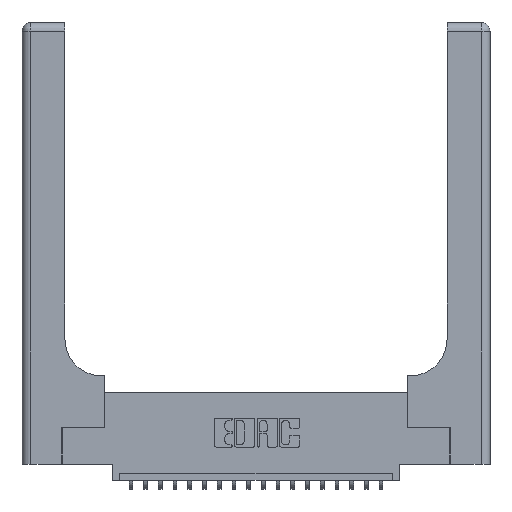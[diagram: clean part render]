
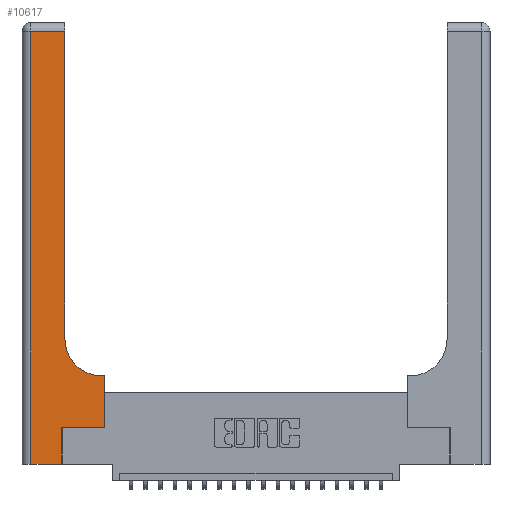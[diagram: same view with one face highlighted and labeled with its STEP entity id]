
A CAD part, top view. The second image highlights one B-rep face of the part: STEP entity #10617.
In plain terms, the highlighted planar face has unit normal (0, 0, 1).
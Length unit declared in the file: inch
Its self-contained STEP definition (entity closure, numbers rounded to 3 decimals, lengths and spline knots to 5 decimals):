
#414 = CARTESIAN_POINT ( 'NONE',  ( 0.2915, 0.85, 0.37 ) ) ;
#464 = CARTESIAN_POINT ( 'NONE',  ( 0., 3., 0.37 ) ) ;
#840 = VERTEX_POINT ( 'NONE', #6834 ) ;
#920 = VERTEX_POINT ( 'NONE', #7125 ) ;
#981 = EDGE_CURVE ( 'NONE', #17231, #18543, #9277, .T. ) ;
#1384 = EDGE_CURVE ( 'NONE', #18543, #18595, #11652, .T. ) ;
#2075 = CARTESIAN_POINT ( 'NONE',  ( 0.5415, 0.85, 0.37 ) ) ;
#2097 = CARTESIAN_POINT ( 'NONE',  ( 0.269, 0., 0.37 ) ) ;
#2369 = DIRECTION ( 'NONE',  ( 0., 1., 0. ) ) ;
#2375 = PLANE ( 'NONE',  #16137 ) ;
#2440 = EDGE_CURVE ( 'NONE', #20743, #15297, #5850, .T. ) ;
#2452 = AXIS2_PLACEMENT_3D ( 'NONE', #2075, #9241, #14116 ) ;
#2867 = VECTOR ( 'NONE', #17015, 39.37008 ) ;
#3347 = CARTESIAN_POINT ( 'NONE',  ( 0.269, 0., 0.37 ) ) ;
#3706 = ORIENTED_EDGE ( 'NONE', *, *, #5183, .T. ) ;
#4435 = DIRECTION ( 'NONE',  ( -1., 0., 0. ) ) ;
#5088 = DIRECTION ( 'NONE',  ( 0., 1., 0. ) ) ;
#5183 = EDGE_CURVE ( 'NONE', #18595, #920, #20500, .T. ) ;
#5621 = CARTESIAN_POINT ( 'NONE',  ( 0.5585, 0.25, 0.37 ) ) ;
#5692 = DIRECTION ( 'NONE',  ( 1., 0., 0. ) ) ;
#5848 = ORIENTED_EDGE ( 'NONE', *, *, #1384, .T. ) ;
#5850 = LINE ( 'NONE', #12152, #2867 ) ;
#6146 = EDGE_CURVE ( 'NONE', #12673, #20743, #8691, .T. ) ;
#6770 = VECTOR ( 'NONE', #2369, 39.37008 ) ;
#6834 = CARTESIAN_POINT ( 'NONE',  ( 0.06, 0., 0.37 ) ) ;
#7125 = CARTESIAN_POINT ( 'NONE',  ( 0.06, 2.94, 0.37 ) ) ;
#7727 = DIRECTION ( 'NONE',  ( -1., 0., 0. ) ) ;
#7794 = EDGE_CURVE ( 'NONE', #840, #12673, #11014, .T. ) ;
#7900 = EDGE_CURVE ( 'NONE', #18801, #17231, #8887, .T. ) ;
#7973 = ORIENTED_EDGE ( 'NONE', *, *, #7794, .T. ) ;
#8425 = CARTESIAN_POINT ( 'NONE',  ( 0.5415, 0.6, 0.37 ) ) ;
#8691 = LINE ( 'NONE', #3347, #17261 ) ;
#8799 = ORIENTED_EDGE ( 'NONE', *, *, #981, .T. ) ;
#8887 = LINE ( 'NONE', #19068, #13973 ) ;
#9241 = DIRECTION ( 'NONE',  ( 0., 0., -1. ) ) ;
#9277 = CIRCLE ( 'NONE', #2452, 0.25 ) ;
#9491 = CARTESIAN_POINT ( 'NONE',  ( 0.2915, 3., 0.37 ) ) ;
#10617 = ADVANCED_FACE ( 'NONE', ( #17557 ), #2375, .F. ) ;
#10801 = ORIENTED_EDGE ( 'NONE', *, *, #11058, .T. ) ;
#10949 = ORIENTED_EDGE ( 'NONE', *, *, #16223, .T. ) ;
#11014 = LINE ( 'NONE', #14267, #18786 ) ;
#11058 = EDGE_CURVE ( 'NONE', #920, #840, #20718, .T. ) ;
#11112 = CARTESIAN_POINT ( 'NONE',  ( 0., 2.94, 0.37 ) ) ;
#11652 = LINE ( 'NONE', #9491, #15432 ) ;
#12152 = CARTESIAN_POINT ( 'NONE',  ( 0.269, 0.25, 0.37 ) ) ;
#12153 = CARTESIAN_POINT ( 'NONE',  ( 0.06, 3., 0.37 ) ) ;
#12433 = DIRECTION ( 'NONE',  ( 0., -1., 0. ) ) ;
#12541 = DIRECTION ( 'NONE',  ( 0., 0., -1. ) ) ;
#12673 = VERTEX_POINT ( 'NONE', #2097 ) ;
#13475 = VECTOR ( 'NONE', #12433, 39.37008 ) ;
#13973 = VECTOR ( 'NONE', #4435, 39.37008 ) ;
#14116 = DIRECTION ( 'NONE',  ( 1., 0., 0. ) ) ;
#14267 = CARTESIAN_POINT ( 'NONE',  ( 0., 0., 0.37 ) ) ;
#15297 = VERTEX_POINT ( 'NONE', #16690 ) ;
#15432 = VECTOR ( 'NONE', #17931, 39.37008 ) ;
#15659 = LINE ( 'NONE', #5621, #6770 ) ;
#15987 = VECTOR ( 'NONE', #7727, 39.37008 ) ;
#16137 = AXIS2_PLACEMENT_3D ( 'NONE', #464, #12541, #19272 ) ;
#16223 = EDGE_CURVE ( 'NONE', #15297, #18801, #15659, .T. ) ;
#16407 = CARTESIAN_POINT ( 'NONE',  ( 0.269, 0.25, 0.37 ) ) ;
#16690 = CARTESIAN_POINT ( 'NONE',  ( 0.5585, 0.25, 0.37 ) ) ;
#17015 = DIRECTION ( 'NONE',  ( 1., 0., 0. ) ) ;
#17231 = VERTEX_POINT ( 'NONE', #8425 ) ;
#17261 = VECTOR ( 'NONE', #5088, 39.37008 ) ;
#17508 = ORIENTED_EDGE ( 'NONE', *, *, #6146, .T. ) ;
#17557 = FACE_OUTER_BOUND ( 'NONE', #21991, .T. ) ;
#17931 = DIRECTION ( 'NONE',  ( 0., 1., 0. ) ) ;
#18192 = ORIENTED_EDGE ( 'NONE', *, *, #7900, .T. ) ;
#18230 = ORIENTED_EDGE ( 'NONE', *, *, #2440, .T. ) ;
#18543 = VERTEX_POINT ( 'NONE', #414 ) ;
#18595 = VERTEX_POINT ( 'NONE', #19224 ) ;
#18786 = VECTOR ( 'NONE', #5692, 39.37008 ) ;
#18801 = VERTEX_POINT ( 'NONE', #21729 ) ;
#19068 = CARTESIAN_POINT ( 'NONE',  ( 0.2915, 0.6, 0.37 ) ) ;
#19224 = CARTESIAN_POINT ( 'NONE',  ( 0.2915, 2.94, 0.37 ) ) ;
#19272 = DIRECTION ( 'NONE',  ( -1., 0., 0. ) ) ;
#20500 = LINE ( 'NONE', #11112, #15987 ) ;
#20718 = LINE ( 'NONE', #12153, #13475 ) ;
#20743 = VERTEX_POINT ( 'NONE', #16407 ) ;
#21729 = CARTESIAN_POINT ( 'NONE',  ( 0.5585, 0.6, 0.37 ) ) ;
#21991 = EDGE_LOOP ( 'NONE', ( #5848, #3706, #10801, #7973, #17508, #18230, #10949, #18192, #8799 ) ) ;
